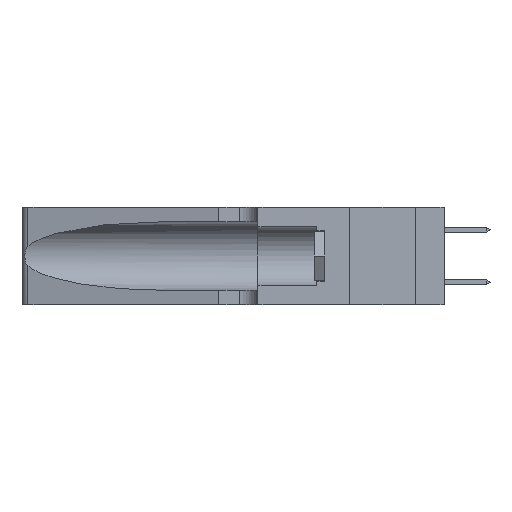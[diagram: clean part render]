
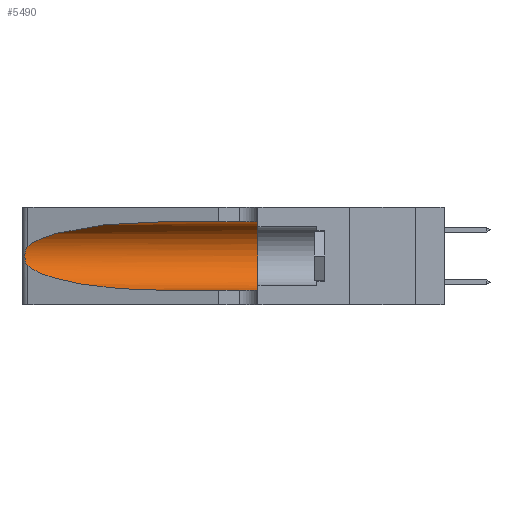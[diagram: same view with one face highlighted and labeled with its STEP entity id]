
A CAD part, left-side view. The second image highlights one B-rep face of the part: STEP entity #5490.
In plain terms, the highlighted cylindrical face has radius 3.308 mm (diameter 6.617 mm), a partial arc.
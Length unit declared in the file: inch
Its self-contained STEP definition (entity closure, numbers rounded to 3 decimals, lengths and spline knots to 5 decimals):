
#729 = AXIS2_PLACEMENT_3D ( 'NONE', #16148, #5427, #17909 ) ;
#759 = CARTESIAN_POINT ( 'NONE',  ( 0.1305, 0.35, 0.05475 ) ) ;
#765 = ORIENTED_EDGE ( 'NONE', *, *, #21363, .T. ) ;
#1080 = CARTESIAN_POINT ( 'NONE',  ( 0.25487, 1.22718, 0.22369 ) ) ;
#1466 = CARTESIAN_POINT ( 'NONE',  ( 0.1305, 1.61858, 0.185 ) ) ;
#1538 = CARTESIAN_POINT ( 'NONE',  ( 0.18966, 0.96281, 0.05475 ) ) ;
#1638 = CARTESIAN_POINT ( 'NONE',  ( 0.25555, 1.22994, 0.2215 ) ) ;
#2070 = CARTESIAN_POINT ( 'NONE',  ( 0.1305, 1.61858, 0.31525 ) ) ;
#2979 = CYLINDRICAL_SURFACE ( 'NONE', #4006, 0.13025 ) ;
#3463 = CARTESIAN_POINT ( 'NONE',  ( 0.25787, 1.23484, 0.2124 ) ) ;
#3659 = CARTESIAN_POINT ( 'NONE',  ( 0.1305, 0.72297, 0.05475 ) ) ;
#3936 = ORIENTED_EDGE ( 'NONE', *, *, #9110, .T. ) ;
#4006 = AXIS2_PLACEMENT_3D ( 'NONE', #1466, #14071, #12309 ) ;
#4483 = VECTOR ( 'NONE', #12492, 39.37008 ) ;
#4654 = CARTESIAN_POINT ( 'NONE',  ( 0.1305, 0.72297, 0.31525 ) ) ;
#5280 = CARTESIAN_POINT ( 'NONE',  ( 0.26018, 1.23835, 0.19895 ) ) ;
#5427 = DIRECTION ( 'NONE',  ( 0., 1., 0. ) ) ;
#5490 = ADVANCED_FACE ( 'NONE', ( #17247 ), #2979, .F. ) ;
#6895 = EDGE_LOOP ( 'NONE', ( #765, #7875, #11061, #3936, #21728, #19850 ) ) ;
#6952 = VERTEX_POINT ( 'NONE', #759 ) ;
#7092 = CARTESIAN_POINT ( 'NONE',  ( 0.26075, 1.23896, 0.178 ) ) ;
#7875 = ORIENTED_EDGE ( 'NONE', *, *, #21533, .T. ) ;
#7908 = LINE ( 'NONE', #2070, #16823 ) ;
#7985 = VERTEX_POINT ( 'NONE', #3659 ) ;
#8754 = CARTESIAN_POINT ( 'NONE',  ( 0.25487, 1.22718, 0.14631 ) ) ;
#8932 = CARTESIAN_POINT ( 'NONE',  ( 0.25856, 1.23593, 0.16098 ) ) ;
#9110 = EDGE_CURVE ( 'NONE', #7985, #6952, #13525, .T. ) ;
#10804 = CARTESIAN_POINT ( 'NONE',  ( 0.25639, 1.23186, 0.15144 ) ) ;
#11061 = ORIENTED_EDGE ( 'NONE', *, *, #14354, .T. ) ;
#11828 = EDGE_CURVE ( 'NONE', #15719, #6952, #19050, .T. ) ;
#11946 = CARTESIAN_POINT ( 'NONE',  ( 0.2373, 1.15595, 0.28018 ) ) ;
#12309 = DIRECTION ( 'NONE',  ( 0., 0., -1. ) ) ;
#12492 = DIRECTION ( 'NONE',  ( 0., -1., 0. ) ) ;
#12559 = CARTESIAN_POINT ( 'NONE',  ( 0.25487, 1.22718, 0.14631 ) ) ;
#13525 = LINE ( 'NONE', #22900, #4483 ) ;
#14071 = DIRECTION ( 'NONE',  ( 0., -1., 0. ) ) ;
#14148 = CARTESIAN_POINT ( 'NONE',  ( 0.1305, 0.72297, 0.05475 ) ) ;
#14248 = CARTESIAN_POINT ( 'NONE',  ( 0.25639, 1.23184, 0.21858 ) ) ;
#14286 = B_SPLINE_CURVE_WITH_KNOTS ( 'NONE', 3,
 ( #22886, #1638, #14248, #3463, #16000, #5280, #17766, #7092, #19515, #8932, #21228, #10804, #22960, #12559 ),
 .UNSPECIFIED., .F., .F.,
 ( 4, 2, 2, 2, 2, 2, 4 ),
 ( 0., 0.00027, 0.00053, 0.00107, 0.0016, 0.00187, 0.00214 ),
 .UNSPECIFIED. ) ;
#14354 = EDGE_CURVE ( 'NONE', #22513, #7985, #15956, .T. ) ;
#15651 = VERTEX_POINT ( 'NONE', #19989 ) ;
#15719 = VERTEX_POINT ( 'NONE', #16738 ) ;
#15956 =( BOUNDED_CURVE ( )  B_SPLINE_CURVE ( 3, ( #8754, #19348, #1538, #14148 ),
 .UNSPECIFIED., .F., .T. ) 
 B_SPLINE_CURVE_WITH_KNOTS ( ( 4, 4 ),
 ( 3.44316, 4.71239 ),
 .UNSPECIFIED. ) 
 CURVE ( )  GEOMETRIC_REPRESENTATION_ITEM ( )  RATIONAL_B_SPLINE_CURVE ( ( 1., 0.87, 0.87, 1. ) ) 
 REPRESENTATION_ITEM ( '' )  );
#16000 = CARTESIAN_POINT ( 'NONE',  ( 0.25854, 1.2359, 0.20912 ) ) ;
#16148 = CARTESIAN_POINT ( 'NONE',  ( 0.1305, 0.35, 0.185 ) ) ;
#16411 = DIRECTION ( 'NONE',  ( 0., -1., 0. ) ) ;
#16738 = CARTESIAN_POINT ( 'NONE',  ( 0.1305, 0.35, 0.31525 ) ) ;
#16823 = VECTOR ( 'NONE', #16411, 39.37008 ) ;
#17247 = FACE_OUTER_BOUND ( 'NONE', #6895, .T. ) ;
#17604 = EDGE_CURVE ( 'NONE', #15651, #15719, #7908, .T. ) ;
#17766 = CARTESIAN_POINT ( 'NONE',  ( 0.26075, 1.23896, 0.19203 ) ) ;
#17909 = DIRECTION ( 'NONE',  ( 0., 0., 1. ) ) ;
#18337 =( BOUNDED_CURVE ( )  B_SPLINE_CURVE ( 3, ( #4654, #20626, #11946, #1080 ),
 .UNSPECIFIED., .F., .T. ) 
 B_SPLINE_CURVE_WITH_KNOTS ( ( 4, 4 ),
 ( 1.5708, 2.84003 ),
 .UNSPECIFIED. ) 
 CURVE ( )  GEOMETRIC_REPRESENTATION_ITEM ( )  RATIONAL_B_SPLINE_CURVE ( ( 1., 0.87, 0.87, 1. ) ) 
 REPRESENTATION_ITEM ( '' )  );
#19050 = CIRCLE ( 'NONE', #729, 0.13025 ) ;
#19346 = CARTESIAN_POINT ( 'NONE',  ( 0.25487, 1.22718, 0.22369 ) ) ;
#19348 = CARTESIAN_POINT ( 'NONE',  ( 0.2373, 1.15595, 0.08982 ) ) ;
#19515 = CARTESIAN_POINT ( 'NONE',  ( 0.26017, 1.23833, 0.17102 ) ) ;
#19850 = ORIENTED_EDGE ( 'NONE', *, *, #17604, .F. ) ;
#19989 = CARTESIAN_POINT ( 'NONE',  ( 0.1305, 0.72297, 0.31525 ) ) ;
#20133 = CARTESIAN_POINT ( 'NONE',  ( 0.25487, 1.22718, 0.14631 ) ) ;
#20503 = VERTEX_POINT ( 'NONE', #19346 ) ;
#20626 = CARTESIAN_POINT ( 'NONE',  ( 0.18966, 0.96281, 0.31525 ) ) ;
#21228 = CARTESIAN_POINT ( 'NONE',  ( 0.25789, 1.23486, 0.15765 ) ) ;
#21363 = EDGE_CURVE ( 'NONE', #15651, #20503, #18337, .T. ) ;
#21533 = EDGE_CURVE ( 'NONE', #20503, #22513, #14286, .T. ) ;
#21728 = ORIENTED_EDGE ( 'NONE', *, *, #11828, .F. ) ;
#22513 = VERTEX_POINT ( 'NONE', #20133 ) ;
#22886 = CARTESIAN_POINT ( 'NONE',  ( 0.25487, 1.22718, 0.22369 ) ) ;
#22900 = CARTESIAN_POINT ( 'NONE',  ( 0.1305, 1.61858, 0.05475 ) ) ;
#22960 = CARTESIAN_POINT ( 'NONE',  ( 0.25555, 1.22993, 0.14849 ) ) ;
